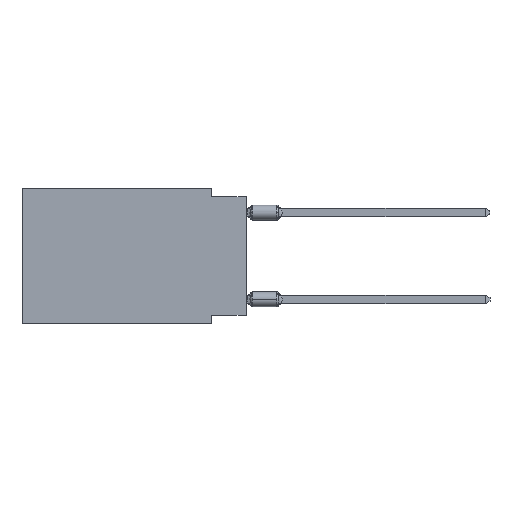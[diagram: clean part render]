
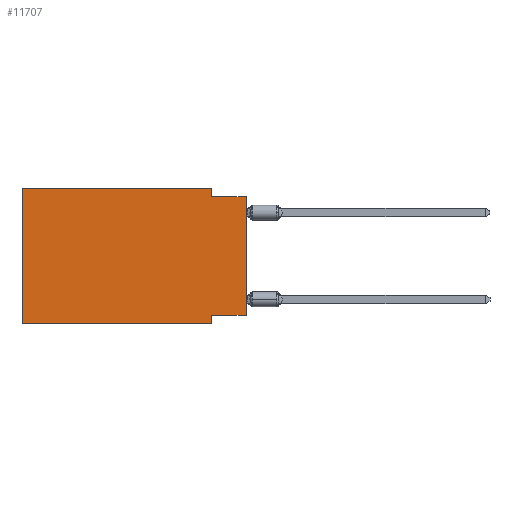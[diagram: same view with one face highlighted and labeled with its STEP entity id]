
A CAD part, left-side view. The second image highlights one B-rep face of the part: STEP entity #11707.
In plain terms, the highlighted planar face has unit normal (-1, 0, 0).
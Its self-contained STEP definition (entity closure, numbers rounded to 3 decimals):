
#7 = CARTESIAN_POINT ( 'NONE',  ( 0., 0., 0. ) ) ;
#203 = VERTEX_POINT ( 'NONE', #1538 ) ;
#559 = CARTESIAN_POINT ( 'NONE',  ( 0., 0., -0.635 ) ) ;
#930 = EDGE_CURVE ( 'NONE', #15544, #10936, #15492, .T. ) ;
#1098 = EDGE_CURVE ( 'NONE', #12076, #11784, #6802, .T. ) ;
#1159 = LINE ( 'NONE', #11674, #7148 ) ;
#1325 = LINE ( 'NONE', #7, #11010 ) ;
#1481 = ORIENTED_EDGE ( 'NONE', *, *, #3884, .T. ) ;
#1538 = CARTESIAN_POINT ( 'NONE',  ( 0., 16.383, 0. ) ) ;
#2228 = VECTOR ( 'NONE', #15362, 1000. ) ;
#3060 = LINE ( 'NONE', #9685, #6790 ) ;
#3193 = DIRECTION ( 'NONE',  ( 1., 0., 0. ) ) ;
#3311 = DIRECTION ( 'NONE',  ( 0., -1., 0. ) ) ;
#3345 = ORIENTED_EDGE ( 'NONE', *, *, #11851, .F. ) ;
#3506 = ORIENTED_EDGE ( 'NONE', *, *, #16395, .F. ) ;
#3800 = CARTESIAN_POINT ( 'NONE',  ( 0., 2.54, -9.906 ) ) ;
#3884 = EDGE_CURVE ( 'NONE', #15544, #7200, #1325, .T. ) ;
#4592 = VECTOR ( 'NONE', #15402, 1000. ) ;
#4796 = CARTESIAN_POINT ( 'NONE',  ( 0., 0., -9.271 ) ) ;
#5241 = DIRECTION ( 'NONE',  ( 0., 0., -1. ) ) ;
#5347 = ORIENTED_EDGE ( 'NONE', *, *, #1098, .T. ) ;
#5728 = DIRECTION ( 'NONE',  ( 0., 0., -1. ) ) ;
#5847 = DIRECTION ( 'NONE',  ( 0., -1., 0. ) ) ;
#6606 = EDGE_CURVE ( 'NONE', #10936, #11784, #12161, .T. ) ;
#6790 = VECTOR ( 'NONE', #3311, 1000. ) ;
#6802 = LINE ( 'NONE', #13164, #8740 ) ;
#7118 = CARTESIAN_POINT ( 'NONE',  ( 0., 16.383, 0. ) ) ;
#7148 = VECTOR ( 'NONE', #5241, 1000. ) ;
#7200 = VERTEX_POINT ( 'NONE', #13783 ) ;
#7216 = AXIS2_PLACEMENT_3D ( 'NONE', #7118, #3193, #5728 ) ;
#7525 = CARTESIAN_POINT ( 'NONE',  ( 0., 16.383, 0. ) ) ;
#8063 = ORIENTED_EDGE ( 'NONE', *, *, #16818, .F. ) ;
#8740 = VECTOR ( 'NONE', #12120, 1000. ) ;
#9629 = CARTESIAN_POINT ( 'NONE',  ( 0., 2.54, -9.906 ) ) ;
#9685 = CARTESIAN_POINT ( 'NONE',  ( 0., 16.383, 0. ) ) ;
#9803 = CARTESIAN_POINT ( 'NONE',  ( 0., 16.383, -9.906 ) ) ;
#10073 = LINE ( 'NONE', #7525, #2228 ) ;
#10155 = CARTESIAN_POINT ( 'NONE',  ( 0., 2.54, -0.635 ) ) ;
#10543 = VERTEX_POINT ( 'NONE', #12269 ) ;
#10608 = VECTOR ( 'NONE', #13809, 1000. ) ;
#10711 = DIRECTION ( 'NONE',  ( 0., 0., 1. ) ) ;
#10936 = VERTEX_POINT ( 'NONE', #13387 ) ;
#11010 = VECTOR ( 'NONE', #10711, 1000. ) ;
#11296 = FACE_OUTER_BOUND ( 'NONE', #15015, .T. ) ;
#11674 = CARTESIAN_POINT ( 'NONE',  ( 0., 2.54, 0. ) ) ;
#11707 = ADVANCED_FACE ( 'NONE', ( #11296 ), #13658, .F. ) ;
#11784 = VERTEX_POINT ( 'NONE', #3800 ) ;
#11812 = VERTEX_POINT ( 'NONE', #10155 ) ;
#11851 = EDGE_CURVE ( 'NONE', #12076, #203, #10073, .T. ) ;
#12076 = VERTEX_POINT ( 'NONE', #9803 ) ;
#12120 = DIRECTION ( 'NONE',  ( 0., -1., 0. ) ) ;
#12161 = LINE ( 'NONE', #9629, #10608 ) ;
#12269 = CARTESIAN_POINT ( 'NONE',  ( 0., 2.54, 0. ) ) ;
#12293 = CARTESIAN_POINT ( 'NONE',  ( 0., 0., -9.271 ) ) ;
#12484 = LINE ( 'NONE', #559, #16197 ) ;
#12740 = EDGE_CURVE ( 'NONE', #10543, #11812, #1159, .T. ) ;
#13164 = CARTESIAN_POINT ( 'NONE',  ( 0., 16.383, -9.906 ) ) ;
#13387 = CARTESIAN_POINT ( 'NONE',  ( 0., 2.54, -9.271 ) ) ;
#13658 = PLANE ( 'NONE',  #7216 ) ;
#13783 = CARTESIAN_POINT ( 'NONE',  ( 0., 0., -0.635 ) ) ;
#13809 = DIRECTION ( 'NONE',  ( 0., 0., -1. ) ) ;
#14016 = ORIENTED_EDGE ( 'NONE', *, *, #12740, .F. ) ;
#15015 = EDGE_LOOP ( 'NONE', ( #1481, #3506, #14016, #8063, #3345, #5347, #15400, #16273 ) ) ;
#15362 = DIRECTION ( 'NONE',  ( 0., 0., 1. ) ) ;
#15400 = ORIENTED_EDGE ( 'NONE', *, *, #6606, .F. ) ;
#15402 = DIRECTION ( 'NONE',  ( 0., 1., 0. ) ) ;
#15492 = LINE ( 'NONE', #4796, #4592 ) ;
#15544 = VERTEX_POINT ( 'NONE', #12293 ) ;
#16197 = VECTOR ( 'NONE', #5847, 1000. ) ;
#16273 = ORIENTED_EDGE ( 'NONE', *, *, #930, .F. ) ;
#16395 = EDGE_CURVE ( 'NONE', #11812, #7200, #12484, .T. ) ;
#16818 = EDGE_CURVE ( 'NONE', #203, #10543, #3060, .T. ) ;
